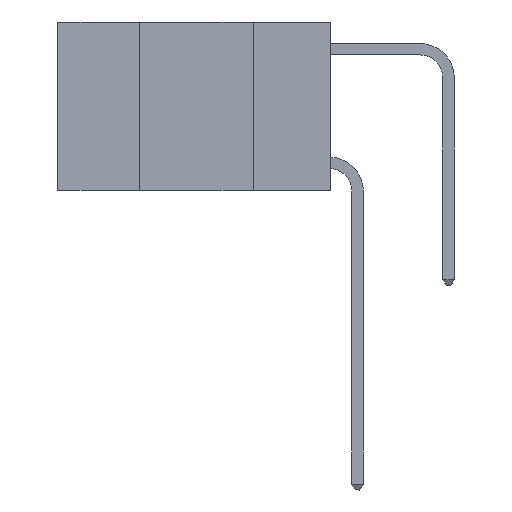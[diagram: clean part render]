
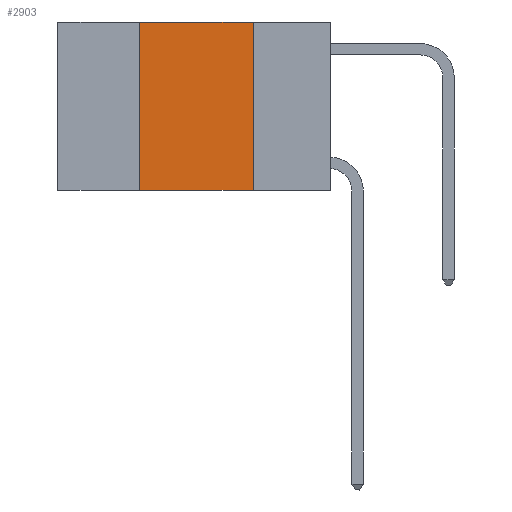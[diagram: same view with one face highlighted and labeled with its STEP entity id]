
A CAD part, left-side view. The second image highlights one B-rep face of the part: STEP entity #2903.
In plain terms, the highlighted planar face has unit normal (-1, 0, 0).
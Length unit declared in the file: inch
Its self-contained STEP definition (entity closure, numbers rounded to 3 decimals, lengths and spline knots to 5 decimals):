
#177 = EDGE_CURVE ( 'NONE', #6065, #10553, #207, .T. ) ;
#207 = LINE ( 'NONE', #10681, #2465 ) ;
#255 = CARTESIAN_POINT ( 'NONE',  ( 0., 0.42, 0. ) ) ;
#399 = FACE_OUTER_BOUND ( 'NONE', #1163, .T. ) ;
#1163 = EDGE_LOOP ( 'NONE', ( #9552, #7164, #6559, #4336 ) ) ;
#1642 = CARTESIAN_POINT ( 'NONE',  ( 0., 0.6, 0. ) ) ;
#2057 = DIRECTION ( 'NONE',  ( 0., 0., 1. ) ) ;
#2465 = VECTOR ( 'NONE', #8207, 39.37008 ) ;
#2903 = ADVANCED_FACE ( 'NONE', ( #399 ), #8305, .F. ) ;
#3397 = DIRECTION ( 'NONE',  ( 0., -1., 0. ) ) ;
#3398 = DIRECTION ( 'NONE',  ( 0., 0., -1. ) ) ;
#3749 = CARTESIAN_POINT ( 'NONE',  ( 0., 0.42, -0.37 ) ) ;
#4190 = DIRECTION ( 'NONE',  ( 0., -1., 0. ) ) ;
#4200 = DIRECTION ( 'NONE',  ( 1., 0., 0. ) ) ;
#4336 = ORIENTED_EDGE ( 'NONE', *, *, #5086, .T. ) ;
#4389 = AXIS2_PLACEMENT_3D ( 'NONE', #1642, #4200, #3398 ) ;
#4490 = LINE ( 'NONE', #9179, #6683 ) ;
#4860 = VERTEX_POINT ( 'NONE', #3749 ) ;
#4878 = EDGE_CURVE ( 'NONE', #4860, #8921, #9346, .T. ) ;
#5086 = EDGE_CURVE ( 'NONE', #4860, #10553, #8462, .T. ) ;
#5096 = CARTESIAN_POINT ( 'NONE',  ( 0., 0.17, -0.37 ) ) ;
#6065 = VERTEX_POINT ( 'NONE', #6645 ) ;
#6559 = ORIENTED_EDGE ( 'NONE', *, *, #4878, .F. ) ;
#6562 = CARTESIAN_POINT ( 'NONE',  ( 0., 0.6, -0.37 ) ) ;
#6645 = CARTESIAN_POINT ( 'NONE',  ( 0., 0.17, 0. ) ) ;
#6683 = VECTOR ( 'NONE', #3397, 39.37008 ) ;
#6980 = EDGE_CURVE ( 'NONE', #8921, #6065, #4490, .T. ) ;
#7164 = ORIENTED_EDGE ( 'NONE', *, *, #6980, .F. ) ;
#8207 = DIRECTION ( 'NONE',  ( 0., 0., -1. ) ) ;
#8305 = PLANE ( 'NONE',  #4389 ) ;
#8353 = VECTOR ( 'NONE', #2057, 39.37008 ) ;
#8462 = LINE ( 'NONE', #6562, #8924 ) ;
#8921 = VERTEX_POINT ( 'NONE', #255 ) ;
#8924 = VECTOR ( 'NONE', #4190, 39.37008 ) ;
#9179 = CARTESIAN_POINT ( 'NONE',  ( 0., 0.6, 0. ) ) ;
#9346 = LINE ( 'NONE', #10235, #8353 ) ;
#9552 = ORIENTED_EDGE ( 'NONE', *, *, #177, .F. ) ;
#10235 = CARTESIAN_POINT ( 'NONE',  ( 0., 0.42, 0. ) ) ;
#10553 = VERTEX_POINT ( 'NONE', #5096 ) ;
#10681 = CARTESIAN_POINT ( 'NONE',  ( 0., 0.17, 0. ) ) ;
